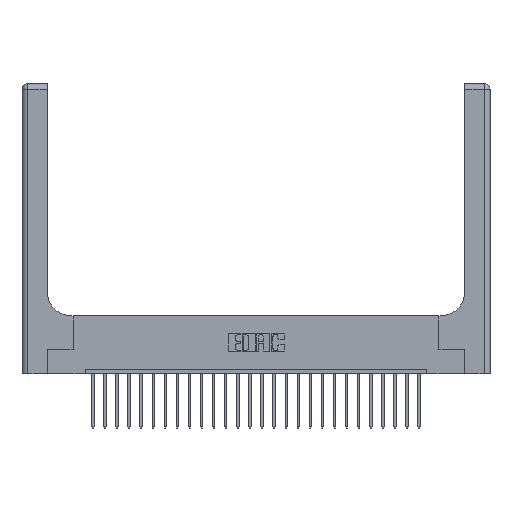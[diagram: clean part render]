
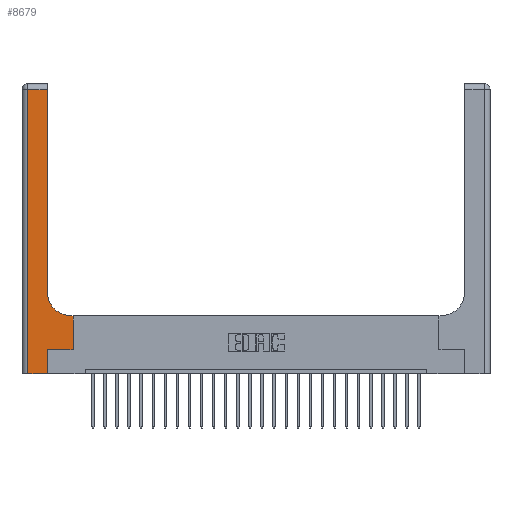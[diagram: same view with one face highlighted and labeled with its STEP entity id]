
A CAD part, top view. The second image highlights one B-rep face of the part: STEP entity #8679.
In plain terms, the highlighted planar face has unit normal (0, 0, 1).
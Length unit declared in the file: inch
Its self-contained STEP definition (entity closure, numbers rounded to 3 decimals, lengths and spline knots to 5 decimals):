
#1008 = EDGE_CURVE ( 'NONE', #20987, #20328, #14922, .T. ) ;
#1104 = CARTESIAN_POINT ( 'NONE',  ( 0.528, 0.6, 0.37 ) ) ;
#1203 = DIRECTION ( 'NONE',  ( 1., 0., 0. ) ) ;
#2887 = DIRECTION ( 'NONE',  ( 0., 0., -1. ) ) ;
#3099 = LINE ( 'NONE', #12668, #4158 ) ;
#3351 = LINE ( 'NONE', #22765, #18633 ) ;
#3428 = CARTESIAN_POINT ( 'NONE',  ( 0.51, 0.6, 0.37 ) ) ;
#4133 = AXIS2_PLACEMENT_3D ( 'NONE', #10034, #14045, #6381 ) ;
#4158 = VECTOR ( 'NONE', #8770, 39.37008 ) ;
#4868 = DIRECTION ( 'NONE',  ( 0., 1., 0. ) ) ;
#5007 = LINE ( 'NONE', #22144, #11727 ) ;
#5115 = ORIENTED_EDGE ( 'NONE', *, *, #22996, .T. ) ;
#5383 = CARTESIAN_POINT ( 'NONE',  ( 0.06, 2.94, 0.37 ) ) ;
#6381 = DIRECTION ( 'NONE',  ( -1., 0., 0. ) ) ;
#7100 = EDGE_CURVE ( 'NONE', #20328, #18713, #15204, .T. ) ;
#7401 = CARTESIAN_POINT ( 'NONE',  ( 0.528, 0.25, 0.37 ) ) ;
#8679 = ADVANCED_FACE ( 'NONE', ( #17946 ), #10161, .F. ) ;
#8764 = CARTESIAN_POINT ( 'NONE',  ( 0.265, 0.25, 0.37 ) ) ;
#8770 = DIRECTION ( 'NONE',  ( 1., 0., 0. ) ) ;
#8826 = CARTESIAN_POINT ( 'NONE',  ( 0.26, 0.6, 0.37 ) ) ;
#9156 = DIRECTION ( 'NONE',  ( 0., 1., 0. ) ) ;
#9288 = CARTESIAN_POINT ( 'NONE',  ( 0.265, 0., 0.37 ) ) ;
#9333 = VECTOR ( 'NONE', #1203, 39.37008 ) ;
#9501 = CARTESIAN_POINT ( 'NONE',  ( 0.26, 2.94, 0.37 ) ) ;
#9600 = DIRECTION ( 'NONE',  ( 0., -1., 0. ) ) ;
#9714 = CARTESIAN_POINT ( 'NONE',  ( 0.06, 3., 0.37 ) ) ;
#10034 = CARTESIAN_POINT ( 'NONE',  ( 0., 3., 0.37 ) ) ;
#10080 = EDGE_CURVE ( 'NONE', #17841, #22578, #10658, .T. ) ;
#10161 = PLANE ( 'NONE',  #4133 ) ;
#10592 = CARTESIAN_POINT ( 'NONE',  ( 0.51, 0.85, 0.37 ) ) ;
#10658 = LINE ( 'NONE', #8764, #9333 ) ;
#11011 = CARTESIAN_POINT ( 'NONE',  ( 0.265, 0.25, 0.37 ) ) ;
#11307 = EDGE_LOOP ( 'NONE', ( #11520, #20965, #5115, #20868, #22799, #15669, #13819, #11574, #23215 ) ) ;
#11520 = ORIENTED_EDGE ( 'NONE', *, *, #1008, .T. ) ;
#11574 = ORIENTED_EDGE ( 'NONE', *, *, #23627, .T. ) ;
#11727 = VECTOR ( 'NONE', #4868, 39.37008 ) ;
#12668 = CARTESIAN_POINT ( 'NONE',  ( 0., 0., 0.37 ) ) ;
#12811 = DIRECTION ( 'NONE',  ( 0., 1., 0. ) ) ;
#12839 = VERTEX_POINT ( 'NONE', #24655 ) ;
#13331 = DIRECTION ( 'NONE',  ( -1., 0., 0. ) ) ;
#13661 = VERTEX_POINT ( 'NONE', #3428 ) ;
#13819 = ORIENTED_EDGE ( 'NONE', *, *, #24701, .T. ) ;
#14045 = DIRECTION ( 'NONE',  ( 0., 0., -1. ) ) ;
#14922 = LINE ( 'NONE', #20259, #18397 ) ;
#15204 = LINE ( 'NONE', #17340, #17731 ) ;
#15669 = ORIENTED_EDGE ( 'NONE', *, *, #10080, .T. ) ;
#16484 = DIRECTION ( 'NONE',  ( -1., 0., 0. ) ) ;
#17251 = LINE ( 'NONE', #9714, #17349 ) ;
#17340 = CARTESIAN_POINT ( 'NONE',  ( 0., 2.94, 0.37 ) ) ;
#17349 = VECTOR ( 'NONE', #9600, 39.37008 ) ;
#17731 = VECTOR ( 'NONE', #13331, 39.37008 ) ;
#17841 = VERTEX_POINT ( 'NONE', #11011 ) ;
#17946 = FACE_OUTER_BOUND ( 'NONE', #11307, .T. ) ;
#18244 = DIRECTION ( 'NONE',  ( 1., 0., 0. ) ) ;
#18397 = VECTOR ( 'NONE', #12811, 39.37008 ) ;
#18633 = VECTOR ( 'NONE', #9156, 39.37008 ) ;
#18713 = VERTEX_POINT ( 'NONE', #5383 ) ;
#20259 = CARTESIAN_POINT ( 'NONE',  ( 0.26, 3., 0.37 ) ) ;
#20328 = VERTEX_POINT ( 'NONE', #9501 ) ;
#20784 = VERTEX_POINT ( 'NONE', #1104 ) ;
#20868 = ORIENTED_EDGE ( 'NONE', *, *, #24705, .T. ) ;
#20965 = ORIENTED_EDGE ( 'NONE', *, *, #7100, .T. ) ;
#20987 = VERTEX_POINT ( 'NONE', #21491 ) ;
#21052 = VECTOR ( 'NONE', #16484, 39.37008 ) ;
#21491 = CARTESIAN_POINT ( 'NONE',  ( 0.26, 0.85, 0.37 ) ) ;
#21821 = AXIS2_PLACEMENT_3D ( 'NONE', #10592, #2887, #18244 ) ;
#21830 = LINE ( 'NONE', #8826, #21052 ) ;
#22144 = CARTESIAN_POINT ( 'NONE',  ( 0.265, 0., 0.37 ) ) ;
#22488 = EDGE_CURVE ( 'NONE', #22553, #17841, #5007, .T. ) ;
#22553 = VERTEX_POINT ( 'NONE', #9288 ) ;
#22578 = VERTEX_POINT ( 'NONE', #7401 ) ;
#22765 = CARTESIAN_POINT ( 'NONE',  ( 0.528, 0.25, 0.37 ) ) ;
#22799 = ORIENTED_EDGE ( 'NONE', *, *, #22488, .T. ) ;
#22996 = EDGE_CURVE ( 'NONE', #18713, #12839, #17251, .T. ) ;
#23201 = EDGE_CURVE ( 'NONE', #13661, #20987, #24231, .T. ) ;
#23215 = ORIENTED_EDGE ( 'NONE', *, *, #23201, .T. ) ;
#23627 = EDGE_CURVE ( 'NONE', #20784, #13661, #21830, .T. ) ;
#24231 = CIRCLE ( 'NONE', #21821, 0.25 ) ;
#24655 = CARTESIAN_POINT ( 'NONE',  ( 0.06, 0., 0.37 ) ) ;
#24701 = EDGE_CURVE ( 'NONE', #22578, #20784, #3351, .T. ) ;
#24705 = EDGE_CURVE ( 'NONE', #12839, #22553, #3099, .T. ) ;
